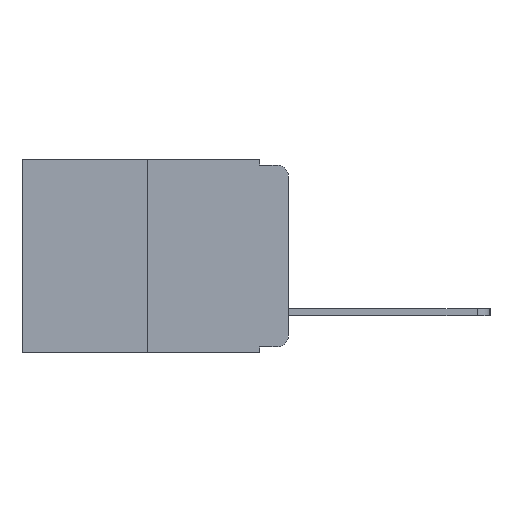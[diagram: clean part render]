
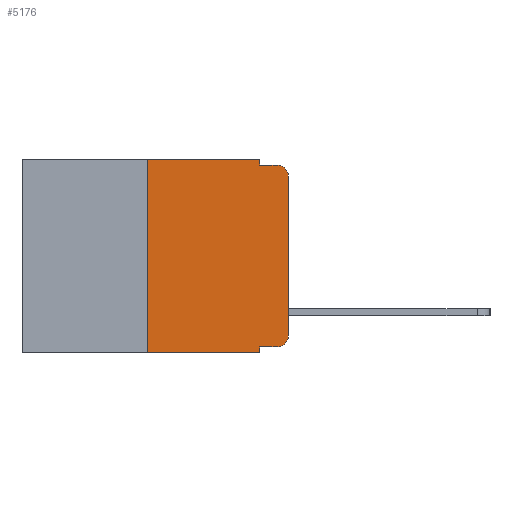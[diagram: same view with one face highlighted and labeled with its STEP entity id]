
A CAD part, left-side view. The second image highlights one B-rep face of the part: STEP entity #5176.
In plain terms, the highlighted planar face has unit normal (-1, 0, 0).
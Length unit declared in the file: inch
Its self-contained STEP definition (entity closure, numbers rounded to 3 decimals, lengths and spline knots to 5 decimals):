
#41 = CARTESIAN_POINT ( 'NONE',  ( 0., 0.25, 0. ) ) ;
#217 = CARTESIAN_POINT ( 'NONE',  ( 0., 0.25, -0.343 ) ) ;
#362 = DIRECTION ( 'NONE',  ( 1., 0., 0. ) ) ;
#376 = AXIS2_PLACEMENT_3D ( 'NONE', #851, #362, #522 ) ;
#473 = PLANE ( 'NONE',  #376 ) ;
#522 = DIRECTION ( 'NONE',  ( 0., 0., -1. ) ) ;
#849 = DIRECTION ( 'NONE',  ( 0., 0., 1. ) ) ;
#851 = CARTESIAN_POINT ( 'NONE',  ( 0., 0.473, 0. ) ) ;
#910 = EDGE_CURVE ( 'NONE', #7989, #9591, #8813, .T. ) ;
#1047 = LINE ( 'NONE', #7937, #3136 ) ;
#1231 = CARTESIAN_POINT ( 'NONE',  ( 0., 0., -0.03 ) ) ;
#1419 = ORIENTED_EDGE ( 'NONE', *, *, #3566, .T. ) ;
#1467 = ORIENTED_EDGE ( 'NONE', *, *, #4716, .F. ) ;
#1890 = AXIS2_PLACEMENT_3D ( 'NONE', #4769, #4801, #4824 ) ;
#1984 = ORIENTED_EDGE ( 'NONE', *, *, #2821, .F. ) ;
#2025 = CARTESIAN_POINT ( 'NONE',  ( 0., 0.051, 0. ) ) ;
#2027 = DIRECTION ( 'NONE',  ( 0., 0., -1. ) ) ;
#2038 = ORIENTED_EDGE ( 'NONE', *, *, #5940, .F. ) ;
#2088 = CARTESIAN_POINT ( 'NONE',  ( 0., 0.473, -0.343 ) ) ;
#2263 = EDGE_CURVE ( 'NONE', #9030, #7989, #12063, .T. ) ;
#2356 = ORIENTED_EDGE ( 'NONE', *, *, #7207, .F. ) ;
#2474 = VECTOR ( 'NONE', #6829, 39.37008 ) ;
#2543 = ORIENTED_EDGE ( 'NONE', *, *, #8426, .T. ) ;
#2821 = EDGE_CURVE ( 'NONE', #4321, #6403, #1047, .T. ) ;
#2844 = DIRECTION ( 'NONE',  ( 0., 0., -1. ) ) ;
#2986 = LINE ( 'NONE', #10451, #9874 ) ;
#3112 = VECTOR ( 'NONE', #2027, 39.37008 ) ;
#3136 = VECTOR ( 'NONE', #8126, 39.37008 ) ;
#3358 = ORIENTED_EDGE ( 'NONE', *, *, #10680, .T. ) ;
#3470 = AXIS2_PLACEMENT_3D ( 'NONE', #5281, #6233, #6660 ) ;
#3490 = EDGE_LOOP ( 'NONE', ( #3358, #2543, #2356, #2038, #1984, #1467, #1419, #5210, #9592, #8934 ) ) ;
#3557 = EDGE_CURVE ( 'NONE', #9030, #4252, #7559, .T. ) ;
#3566 = EDGE_CURVE ( 'NONE', #4342, #4252, #5345, .T. ) ;
#3794 = VECTOR ( 'NONE', #9702, 39.37008 ) ;
#4099 = CARTESIAN_POINT ( 'NONE',  ( 0., 0.02, -0.333 ) ) ;
#4252 = VERTEX_POINT ( 'NONE', #8431 ) ;
#4321 = VERTEX_POINT ( 'NONE', #41 ) ;
#4342 = VERTEX_POINT ( 'NONE', #217 ) ;
#4578 = DIRECTION ( 'NONE',  ( 0., -1., 0. ) ) ;
#4716 = EDGE_CURVE ( 'NONE', #4342, #4321, #6626, .T. ) ;
#4769 = CARTESIAN_POINT ( 'NONE',  ( 0., 0.02, -0.313 ) ) ;
#4787 = VECTOR ( 'NONE', #4578, 39.37008 ) ;
#4801 = DIRECTION ( 'NONE',  ( -1., 0., 0. ) ) ;
#4824 = DIRECTION ( 'NONE',  ( 0., 0., -1. ) ) ;
#4852 = CARTESIAN_POINT ( 'NONE',  ( 0., 0.02, -0.01 ) ) ;
#5176 = ADVANCED_FACE ( 'NONE', ( #7925 ), #473, .F. ) ;
#5210 = ORIENTED_EDGE ( 'NONE', *, *, #3557, .F. ) ;
#5281 = CARTESIAN_POINT ( 'NONE',  ( 0., 0.02, -0.03 ) ) ;
#5345 = LINE ( 'NONE', #2088, #2474 ) ;
#5689 = VERTEX_POINT ( 'NONE', #1231 ) ;
#5940 = EDGE_CURVE ( 'NONE', #6403, #7758, #8629, .T. ) ;
#5967 = LINE ( 'NONE', #6727, #8205 ) ;
#6233 = DIRECTION ( 'NONE',  ( -1., 0., 0. ) ) ;
#6403 = VERTEX_POINT ( 'NONE', #10651 ) ;
#6626 = LINE ( 'NONE', #10036, #3794 ) ;
#6660 = DIRECTION ( 'NONE',  ( 0., 0., -1. ) ) ;
#6727 = CARTESIAN_POINT ( 'NONE',  ( 0., 0., 0. ) ) ;
#6829 = DIRECTION ( 'NONE',  ( 0., -1., 0. ) ) ;
#7207 = EDGE_CURVE ( 'NONE', #7758, #8084, #2986, .T. ) ;
#7559 = LINE ( 'NONE', #2025, #3112 ) ;
#7758 = VERTEX_POINT ( 'NONE', #10765 ) ;
#7925 = FACE_OUTER_BOUND ( 'NONE', #3490, .T. ) ;
#7937 = CARTESIAN_POINT ( 'NONE',  ( 0., 0.473, 0. ) ) ;
#7989 = VERTEX_POINT ( 'NONE', #4099 ) ;
#8084 = VERTEX_POINT ( 'NONE', #4852 ) ;
#8126 = DIRECTION ( 'NONE',  ( 0., -1., 0. ) ) ;
#8205 = VECTOR ( 'NONE', #849, 39.37008 ) ;
#8305 = CIRCLE ( 'NONE', #3470, 0.02 ) ;
#8426 = EDGE_CURVE ( 'NONE', #5689, #8084, #8305, .T. ) ;
#8431 = CARTESIAN_POINT ( 'NONE',  ( 0., 0.051, -0.343 ) ) ;
#8629 = LINE ( 'NONE', #9324, #10159 ) ;
#8813 = CIRCLE ( 'NONE', #1890, 0.02 ) ;
#8934 = ORIENTED_EDGE ( 'NONE', *, *, #910, .T. ) ;
#9030 = VERTEX_POINT ( 'NONE', #11949 ) ;
#9259 = DIRECTION ( 'NONE',  ( 0., -1., 0. ) ) ;
#9324 = CARTESIAN_POINT ( 'NONE',  ( 0., 0.051, 0. ) ) ;
#9591 = VERTEX_POINT ( 'NONE', #9977 ) ;
#9592 = ORIENTED_EDGE ( 'NONE', *, *, #2263, .T. ) ;
#9702 = DIRECTION ( 'NONE',  ( 0., 0., 1. ) ) ;
#9874 = VECTOR ( 'NONE', #9259, 39.37008 ) ;
#9977 = CARTESIAN_POINT ( 'NONE',  ( 0., 0., -0.313 ) ) ;
#10036 = CARTESIAN_POINT ( 'NONE',  ( 0., 0.25, 0. ) ) ;
#10159 = VECTOR ( 'NONE', #2844, 39.37008 ) ;
#10451 = CARTESIAN_POINT ( 'NONE',  ( 0., 0.051, -0.01 ) ) ;
#10651 = CARTESIAN_POINT ( 'NONE',  ( 0., 0.051, 0. ) ) ;
#10680 = EDGE_CURVE ( 'NONE', #9591, #5689, #5967, .T. ) ;
#10765 = CARTESIAN_POINT ( 'NONE',  ( 0., 0.051, -0.01 ) ) ;
#11033 = CARTESIAN_POINT ( 'NONE',  ( 0., 0.051, -0.333 ) ) ;
#11949 = CARTESIAN_POINT ( 'NONE',  ( 0., 0.051, -0.333 ) ) ;
#12063 = LINE ( 'NONE', #11033, #4787 ) ;
